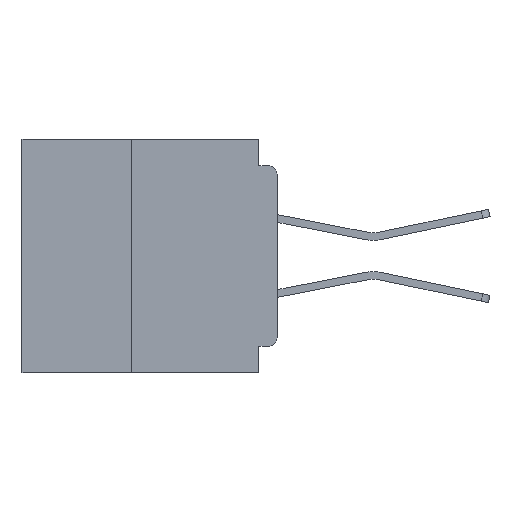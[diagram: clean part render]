
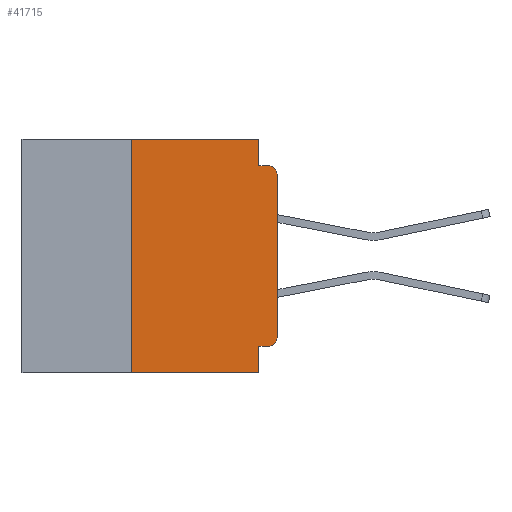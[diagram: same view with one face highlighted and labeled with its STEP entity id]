
A CAD part, left-side view. The second image highlights one B-rep face of the part: STEP entity #41715.
In plain terms, the highlighted planar face has unit normal (-1, 0, 0).
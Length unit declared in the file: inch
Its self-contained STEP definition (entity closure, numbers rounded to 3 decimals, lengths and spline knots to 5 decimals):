
#652 = VERTEX_POINT ( 'NONE', #41814 ) ;
#2489 = VECTOR ( 'NONE', #39236, 39.37008 ) ;
#2730 = VECTOR ( 'NONE', #54040, 39.37008 ) ;
#3098 = EDGE_CURVE ( 'NONE', #58785, #31663, #15387, .T. ) ;
#3348 = CARTESIAN_POINT ( 'NONE',  ( 0., 0.015, -0.355 ) ) ;
#3444 = CARTESIAN_POINT ( 'NONE',  ( 0., 0.25, -0.4 ) ) ;
#3555 = FACE_OUTER_BOUND ( 'NONE', #15345, .T. ) ;
#6062 = CARTESIAN_POINT ( 'NONE',  ( 0., 0., -0.355 ) ) ;
#6470 = EDGE_CURVE ( 'NONE', #652, #58785, #26135, .T. ) ;
#6531 = ORIENTED_EDGE ( 'NONE', *, *, #44482, .F. ) ;
#6836 = ORIENTED_EDGE ( 'NONE', *, *, #3098, .F. ) ;
#7170 = EDGE_CURVE ( 'NONE', #31663, #19229, #9647, .T. ) ;
#7423 = CIRCLE ( 'NONE', #56098, 0.015 ) ;
#8286 = LINE ( 'NONE', #6062, #9845 ) ;
#9647 = LINE ( 'NONE', #39169, #58673 ) ;
#9845 = VECTOR ( 'NONE', #25327, 39.37008 ) ;
#11998 = VECTOR ( 'NONE', #60467, 39.37008 ) ;
#12176 = CARTESIAN_POINT ( 'NONE',  ( 0., 0.015, -0.34 ) ) ;
#13854 = PLANE ( 'NONE',  #45737 ) ;
#14706 = DIRECTION ( 'NONE',  ( -1., 0., 0. ) ) ;
#15345 = EDGE_LOOP ( 'NONE', ( #28901, #20361, #6531, #35197, #6836, #40865, #27940, #24964, #21406, #24907 ) ) ;
#15387 = LINE ( 'NONE', #39227, #2489 ) ;
#17010 = DIRECTION ( 'NONE',  ( 0., 0., -1. ) ) ;
#17689 = VECTOR ( 'NONE', #46141, 39.37008 ) ;
#19229 = VERTEX_POINT ( 'NONE', #20191 ) ;
#20191 = CARTESIAN_POINT ( 'NONE',  ( 0., 0.031, -0.045 ) ) ;
#20361 = ORIENTED_EDGE ( 'NONE', *, *, #32566, .T. ) ;
#21172 = AXIS2_PLACEMENT_3D ( 'NONE', #12176, #45352, #17010 ) ;
#21322 = VERTEX_POINT ( 'NONE', #57817 ) ;
#21406 = ORIENTED_EDGE ( 'NONE', *, *, #61626, .F. ) ;
#22696 = CARTESIAN_POINT ( 'NONE',  ( 0., 0., -0.06 ) ) ;
#23408 = DIRECTION ( 'NONE',  ( 0., 0., -1. ) ) ;
#24529 = EDGE_CURVE ( 'NONE', #58231, #44290, #29650, .T. ) ;
#24907 = ORIENTED_EDGE ( 'NONE', *, *, #52634, .T. ) ;
#24964 = ORIENTED_EDGE ( 'NONE', *, *, #58569, .F. ) ;
#25327 = DIRECTION ( 'NONE',  ( 0., 1., 0. ) ) ;
#26135 = LINE ( 'NONE', #3444, #11998 ) ;
#27940 = ORIENTED_EDGE ( 'NONE', *, *, #53644, .T. ) ;
#28871 = DIRECTION ( 'NONE',  ( 0., -1., 0. ) ) ;
#28901 = ORIENTED_EDGE ( 'NONE', *, *, #24529, .T. ) ;
#28957 = CARTESIAN_POINT ( 'NONE',  ( 0., 0.031, -0.355 ) ) ;
#29650 = LINE ( 'NONE', #30214, #2730 ) ;
#30214 = CARTESIAN_POINT ( 'NONE',  ( 0., 0., 0. ) ) ;
#31663 = VERTEX_POINT ( 'NONE', #31742 ) ;
#31720 = VERTEX_POINT ( 'NONE', #3348 ) ;
#31742 = CARTESIAN_POINT ( 'NONE',  ( 0., 0.031, 0. ) ) ;
#32566 = EDGE_CURVE ( 'NONE', #44290, #37501, #7423, .T. ) ;
#35197 = ORIENTED_EDGE ( 'NONE', *, *, #7170, .F. ) ;
#36977 = CIRCLE ( 'NONE', #21172, 0.015 ) ;
#37501 = VERTEX_POINT ( 'NONE', #38855 ) ;
#37910 = DIRECTION ( 'NONE',  ( 0., -1., 0. ) ) ;
#38855 = CARTESIAN_POINT ( 'NONE',  ( 0., 0.015, -0.045 ) ) ;
#39169 = CARTESIAN_POINT ( 'NONE',  ( 0., 0.031, 0. ) ) ;
#39227 = CARTESIAN_POINT ( 'NONE',  ( 0., 0.437, 0. ) ) ;
#39236 = DIRECTION ( 'NONE',  ( 0., -1., 0. ) ) ;
#40865 = ORIENTED_EDGE ( 'NONE', *, *, #6470, .F. ) ;
#41715 = ADVANCED_FACE ( 'NONE', ( #3555 ), #13854, .F. ) ;
#41814 = CARTESIAN_POINT ( 'NONE',  ( 0., 0.25, -0.4 ) ) ;
#41836 = VERTEX_POINT ( 'NONE', #28957 ) ;
#42882 = LINE ( 'NONE', #56782, #53983 ) ;
#43052 = CARTESIAN_POINT ( 'NONE',  ( 0., 0.015, -0.06 ) ) ;
#44290 = VERTEX_POINT ( 'NONE', #22696 ) ;
#44341 = LINE ( 'NONE', #55686, #17689 ) ;
#44482 = EDGE_CURVE ( 'NONE', #19229, #37501, #57556, .T. ) ;
#45352 = DIRECTION ( 'NONE',  ( -1., 0., 0. ) ) ;
#45737 = AXIS2_PLACEMENT_3D ( 'NONE', #51549, #51766, #23408 ) ;
#46141 = DIRECTION ( 'NONE',  ( 0., 0., -1. ) ) ;
#46418 = VECTOR ( 'NONE', #28871, 39.37008 ) ;
#47821 = DIRECTION ( 'NONE',  ( 0., 0., -1. ) ) ;
#51549 = CARTESIAN_POINT ( 'NONE',  ( 0., 0.437, 0. ) ) ;
#51766 = DIRECTION ( 'NONE',  ( 1., 0., 0. ) ) ;
#52634 = EDGE_CURVE ( 'NONE', #31720, #58231, #36977, .T. ) ;
#53644 = EDGE_CURVE ( 'NONE', #652, #21322, #42882, .T. ) ;
#53983 = VECTOR ( 'NONE', #37910, 39.37008 ) ;
#54040 = DIRECTION ( 'NONE',  ( 0., 0., 1. ) ) ;
#55686 = CARTESIAN_POINT ( 'NONE',  ( 0., 0.031, -0.4 ) ) ;
#56098 = AXIS2_PLACEMENT_3D ( 'NONE', #43052, #14706, #47821 ) ;
#56782 = CARTESIAN_POINT ( 'NONE',  ( 0., 0.437, -0.4 ) ) ;
#56984 = CARTESIAN_POINT ( 'NONE',  ( 0., 0., -0.34 ) ) ;
#57286 = CARTESIAN_POINT ( 'NONE',  ( 0., 0., -0.045 ) ) ;
#57556 = LINE ( 'NONE', #57286, #46418 ) ;
#57817 = CARTESIAN_POINT ( 'NONE',  ( 0., 0.031, -0.4 ) ) ;
#58231 = VERTEX_POINT ( 'NONE', #56984 ) ;
#58259 = DIRECTION ( 'NONE',  ( 0., 0., -1. ) ) ;
#58569 = EDGE_CURVE ( 'NONE', #41836, #21322, #44341, .T. ) ;
#58673 = VECTOR ( 'NONE', #58259, 39.37008 ) ;
#58785 = VERTEX_POINT ( 'NONE', #59867 ) ;
#59867 = CARTESIAN_POINT ( 'NONE',  ( 0., 0.25, 0. ) ) ;
#60467 = DIRECTION ( 'NONE',  ( 0., 0., 1. ) ) ;
#61626 = EDGE_CURVE ( 'NONE', #31720, #41836, #8286, .T. ) ;
